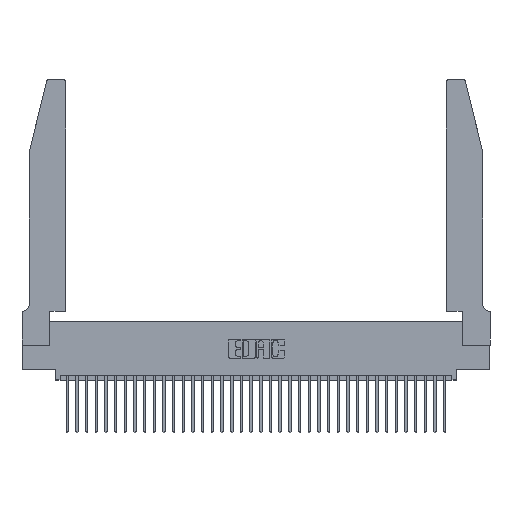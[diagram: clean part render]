
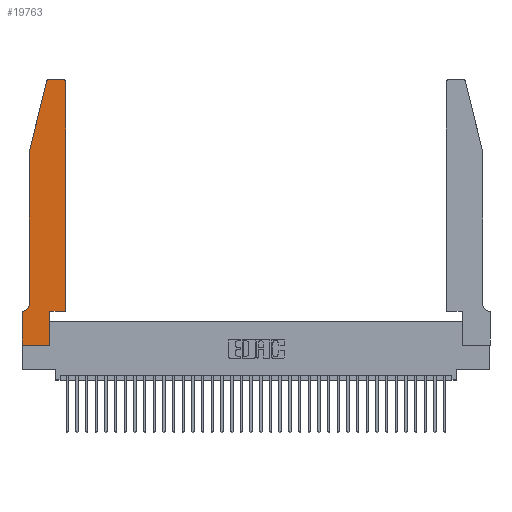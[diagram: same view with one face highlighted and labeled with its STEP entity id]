
A CAD part, top view. The second image highlights one B-rep face of the part: STEP entity #19763.
In plain terms, the highlighted planar face has unit normal (0, 0, 1).
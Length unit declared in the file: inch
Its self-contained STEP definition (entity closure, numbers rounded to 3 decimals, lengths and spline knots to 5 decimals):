
#236 = CARTESIAN_POINT ( 'NONE',  ( 0.0755, 2., 0.37 ) ) ;
#910 = AXIS2_PLACEMENT_3D ( 'NONE', #6680, #26490, #9548 ) ;
#1420 = CARTESIAN_POINT ( 'NONE',  ( 0.0055, 0.35, 0.37 ) ) ;
#1527 = DIRECTION ( 'NONE',  ( 0., -1., 0. ) ) ;
#1668 = CARTESIAN_POINT ( 'NONE',  ( 0.4505, 0.35, 0.37 ) ) ;
#1691 = CIRCLE ( 'NONE', #910, 0.03 ) ;
#2328 = CARTESIAN_POINT ( 'NONE',  ( 0.4205, 2.75, 0.37 ) ) ;
#2571 = ORIENTED_EDGE ( 'NONE', *, *, #24652, .T. ) ;
#2849 = ORIENTED_EDGE ( 'NONE', *, *, #35189, .T. ) ;
#3060 = LINE ( 'NONE', #26875, #8864 ) ;
#3149 = DIRECTION ( 'NONE',  ( 0., -1., 0. ) ) ;
#4364 = ORIENTED_EDGE ( 'NONE', *, *, #28994, .T. ) ;
#4562 = VECTOR ( 'NONE', #14477, 39.37008 ) ;
#5440 = VERTEX_POINT ( 'NONE', #1668 ) ;
#5919 = DIRECTION ( 'NONE',  ( 0., 0., 1. ) ) ;
#6178 = ORIENTED_EDGE ( 'NONE', *, *, #20718, .T. ) ;
#6202 = VERTEX_POINT ( 'NONE', #21878 ) ;
#6680 = CARTESIAN_POINT ( 'NONE',  ( 0.284, 2.72, 0.37 ) ) ;
#6764 = EDGE_CURVE ( 'NONE', #5440, #15830, #30730, .T. ) ;
#6893 = CIRCLE ( 'NONE', #9546, 0.07 ) ;
#7077 = VERTEX_POINT ( 'NONE', #25663 ) ;
#7338 = DIRECTION ( 'NONE',  ( 1., 0., 0. ) ) ;
#7858 = AXIS2_PLACEMENT_3D ( 'NONE', #21481, #24320, #7338 ) ;
#8126 = CARTESIAN_POINT ( 'NONE',  ( 0., 0., 0.37 ) ) ;
#8592 = VERTEX_POINT ( 'NONE', #2328 ) ;
#8864 = VECTOR ( 'NONE', #32410, 39.37008 ) ;
#9319 = VERTEX_POINT ( 'NONE', #26242 ) ;
#9384 = VECTOR ( 'NONE', #32819, 39.37008 ) ;
#9546 = AXIS2_PLACEMENT_3D ( 'NONE', #29062, #12224, #31859 ) ;
#9548 = DIRECTION ( 'NONE',  ( 1., 0., 0. ) ) ;
#9714 = VECTOR ( 'NONE', #22394, 39.37008 ) ;
#9752 = LINE ( 'NONE', #236, #30414 ) ;
#10041 = CARTESIAN_POINT ( 'NONE',  ( 0., 0., 0.37 ) ) ;
#10601 = LINE ( 'NONE', #27416, #9714 ) ;
#11286 = EDGE_CURVE ( 'NONE', #15830, #8592, #26817, .T. ) ;
#11370 = CARTESIAN_POINT ( 'NONE',  ( 0.25487, 2.72718, 0.37 ) ) ;
#11627 = EDGE_LOOP ( 'NONE', ( #2849, #12251, #13208, #4364, #6178, #33043, #2571, #12851, #12430, #31755, #27084, #19621 ) ) ;
#11760 = VERTEX_POINT ( 'NONE', #27764 ) ;
#12224 = DIRECTION ( 'NONE',  ( 0., 0., -1. ) ) ;
#12251 = ORIENTED_EDGE ( 'NONE', *, *, #33753, .T. ) ;
#12430 = ORIENTED_EDGE ( 'NONE', *, *, #33539, .T. ) ;
#12435 = EDGE_CURVE ( 'NONE', #9319, #5440, #27166, .T. ) ;
#12524 = CARTESIAN_POINT ( 'NONE',  ( 0.284, 2.75, 0.37 ) ) ;
#12851 = ORIENTED_EDGE ( 'NONE', *, *, #28089, .T. ) ;
#13161 = DIRECTION ( 'NONE',  ( 0., 1., 0. ) ) ;
#13208 = ORIENTED_EDGE ( 'NONE', *, *, #29380, .T. ) ;
#14477 = DIRECTION ( 'NONE',  ( 1., 0., 0. ) ) ;
#15484 = CARTESIAN_POINT ( 'NONE',  ( 0.2605, 2.75, 0.37 ) ) ;
#15830 = VERTEX_POINT ( 'NONE', #28602 ) ;
#16476 = VECTOR ( 'NONE', #34624, 39.37008 ) ;
#16916 = LINE ( 'NONE', #21603, #9384 ) ;
#17292 = VERTEX_POINT ( 'NONE', #1420 ) ;
#17505 = AXIS2_PLACEMENT_3D ( 'NONE', #22905, #5919, #25747 ) ;
#18583 = VECTOR ( 'NONE', #1527, 39.37008 ) ;
#19621 = ORIENTED_EDGE ( 'NONE', *, *, #11286, .T. ) ;
#19763 = ADVANCED_FACE ( 'NONE', ( #30720 ), #35360, .T. ) ;
#20718 = EDGE_CURVE ( 'NONE', #7077, #17292, #6893, .T. ) ;
#20973 = VERTEX_POINT ( 'NONE', #24486 ) ;
#21481 = CARTESIAN_POINT ( 'NONE',  ( 0., 0.35, 0.37 ) ) ;
#21603 = CARTESIAN_POINT ( 'NONE',  ( 0., 0., 0.37 ) ) ;
#21878 = CARTESIAN_POINT ( 'NONE',  ( 0.2865, 0., 0.37 ) ) ;
#21897 = VERTEX_POINT ( 'NONE', #8126 ) ;
#22394 = DIRECTION ( 'NONE',  ( -0.239, -0.971, 0. ) ) ;
#22905 = CARTESIAN_POINT ( 'NONE',  ( 0.4205, 2.72, 0.37 ) ) ;
#23004 = VERTEX_POINT ( 'NONE', #12524 ) ;
#23355 = VECTOR ( 'NONE', #13161, 39.37008 ) ;
#24034 = LINE ( 'NONE', #26302, #16476 ) ;
#24320 = DIRECTION ( 'NONE',  ( 0., 0., 1. ) ) ;
#24443 = CARTESIAN_POINT ( 'NONE',  ( 0.4505, 0.35, 0.37 ) ) ;
#24486 = CARTESIAN_POINT ( 'NONE',  ( 0.0755, 2., 0.37 ) ) ;
#24652 = EDGE_CURVE ( 'NONE', #11760, #21897, #26088, .T. ) ;
#25663 = CARTESIAN_POINT ( 'NONE',  ( 0.0755, 0.42, 0.37 ) ) ;
#25747 = DIRECTION ( 'NONE',  ( 1., 0., 0. ) ) ;
#25793 = CARTESIAN_POINT ( 'NONE',  ( 0.4505, 0.35, 0.37 ) ) ;
#26088 = LINE ( 'NONE', #10041, #18583 ) ;
#26242 = CARTESIAN_POINT ( 'NONE',  ( 0.2865, 0.35, 0.37 ) ) ;
#26302 = CARTESIAN_POINT ( 'NONE',  ( 0.0755, 0.35, 0.37 ) ) ;
#26490 = DIRECTION ( 'NONE',  ( 0., 0., 1. ) ) ;
#26817 = CIRCLE ( 'NONE', #17505, 0.03 ) ;
#26875 = CARTESIAN_POINT ( 'NONE',  ( 0.2865, 0.35, 0.37 ) ) ;
#27084 = ORIENTED_EDGE ( 'NONE', *, *, #6764, .T. ) ;
#27166 = LINE ( 'NONE', #25793, #4562 ) ;
#27416 = CARTESIAN_POINT ( 'NONE',  ( 0.0755, 2., 0.37 ) ) ;
#27764 = CARTESIAN_POINT ( 'NONE',  ( 0., 0.35, 0.37 ) ) ;
#27864 = EDGE_CURVE ( 'NONE', #17292, #11760, #24034, .T. ) ;
#28089 = EDGE_CURVE ( 'NONE', #21897, #6202, #16916, .T. ) ;
#28602 = CARTESIAN_POINT ( 'NONE',  ( 0.4505, 2.72, 0.37 ) ) ;
#28644 = LINE ( 'NONE', #15484, #36050 ) ;
#28994 = EDGE_CURVE ( 'NONE', #20973, #7077, #9752, .T. ) ;
#29062 = CARTESIAN_POINT ( 'NONE',  ( 0.0055, 0.42, 0.37 ) ) ;
#29380 = EDGE_CURVE ( 'NONE', #34179, #20973, #10601, .T. ) ;
#30414 = VECTOR ( 'NONE', #3149, 39.37008 ) ;
#30720 = FACE_OUTER_BOUND ( 'NONE', #11627, .T. ) ;
#30730 = LINE ( 'NONE', #24443, #23355 ) ;
#31755 = ORIENTED_EDGE ( 'NONE', *, *, #12435, .T. ) ;
#31859 = DIRECTION ( 'NONE',  ( -1., 0., 0. ) ) ;
#32304 = DIRECTION ( 'NONE',  ( -1., 0., 0. ) ) ;
#32410 = DIRECTION ( 'NONE',  ( 0., 1., 0. ) ) ;
#32819 = DIRECTION ( 'NONE',  ( 1., 0., 0. ) ) ;
#33043 = ORIENTED_EDGE ( 'NONE', *, *, #27864, .T. ) ;
#33539 = EDGE_CURVE ( 'NONE', #6202, #9319, #3060, .T. ) ;
#33753 = EDGE_CURVE ( 'NONE', #23004, #34179, #1691, .T. ) ;
#34179 = VERTEX_POINT ( 'NONE', #11370 ) ;
#34624 = DIRECTION ( 'NONE',  ( -1., 0., 0. ) ) ;
#35189 = EDGE_CURVE ( 'NONE', #8592, #23004, #28644, .T. ) ;
#35360 = PLANE ( 'NONE',  #7858 ) ;
#36050 = VECTOR ( 'NONE', #32304, 39.37008 ) ;
